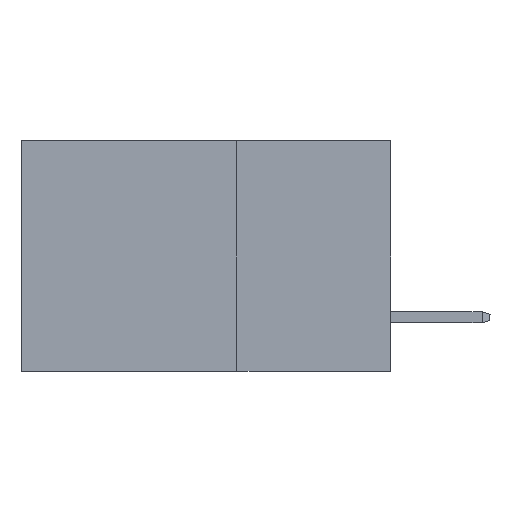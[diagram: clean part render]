
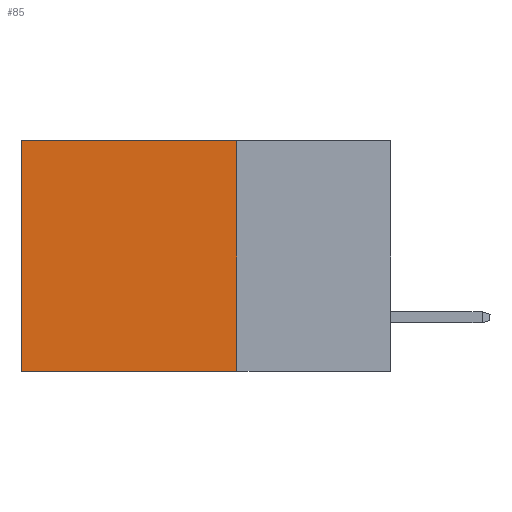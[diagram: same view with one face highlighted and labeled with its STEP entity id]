
A CAD part, left-side view. The second image highlights one B-rep face of the part: STEP entity #85.
In plain terms, the highlighted planar face has unit normal (-1, 0, 0).
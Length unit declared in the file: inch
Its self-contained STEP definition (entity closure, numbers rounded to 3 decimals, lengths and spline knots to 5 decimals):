
#85 = ADVANCED_FACE ( 'NONE', ( #702 ), #11993, .F. ) ;
#434 = VECTOR ( 'NONE', #9236, 39.37008 ) ;
#549 = ORIENTED_EDGE ( 'NONE', *, *, #10817, .F. ) ;
#702 = FACE_OUTER_BOUND ( 'NONE', #3182, .T. ) ;
#765 = ORIENTED_EDGE ( 'NONE', *, *, #3437, .F. ) ;
#810 = LINE ( 'NONE', #1016, #434 ) ;
#1016 = CARTESIAN_POINT ( 'NONE',  ( 0.2875, 0.6, -0.375 ) ) ;
#1050 = EDGE_CURVE ( 'NONE', #3864, #2768, #9512, .T. ) ;
#2768 = VERTEX_POINT ( 'NONE', #12126 ) ;
#3182 = EDGE_LOOP ( 'NONE', ( #14502, #549, #765, #5320 ) ) ;
#3437 = EDGE_CURVE ( 'NONE', #3864, #8057, #5598, .T. ) ;
#3864 = VERTEX_POINT ( 'NONE', #7282 ) ;
#5320 = ORIENTED_EDGE ( 'NONE', *, *, #1050, .T. ) ;
#5343 = EDGE_CURVE ( 'NONE', #2768, #10095, #810, .T. ) ;
#5598 = LINE ( 'NONE', #13385, #8169 ) ;
#6017 = DIRECTION ( 'NONE',  ( 0., 0., -1. ) ) ;
#6789 = CARTESIAN_POINT ( 'NONE',  ( 0.2875, 0.6, -0.375 ) ) ;
#7028 = CARTESIAN_POINT ( 'NONE',  ( 0.2875, 0.25, -0.375 ) ) ;
#7282 = CARTESIAN_POINT ( 'NONE',  ( 0.2875, 0.25, 0. ) ) ;
#7351 = VECTOR ( 'NONE', #8537, 39.37008 ) ;
#8057 = VERTEX_POINT ( 'NONE', #7028 ) ;
#8169 = VECTOR ( 'NONE', #13486, 39.37008 ) ;
#8257 = VECTOR ( 'NONE', #13772, 39.37008 ) ;
#8514 = CARTESIAN_POINT ( 'NONE',  ( 0.2875, 0.25, -0.375 ) ) ;
#8537 = DIRECTION ( 'NONE',  ( 0., 1., 0. ) ) ;
#8634 = CARTESIAN_POINT ( 'NONE',  ( 0.2875, 0.25, -0.375 ) ) ;
#9236 = DIRECTION ( 'NONE',  ( 0., 0., -1. ) ) ;
#9512 = LINE ( 'NONE', #11329, #8257 ) ;
#10095 = VERTEX_POINT ( 'NONE', #6789 ) ;
#10643 = DIRECTION ( 'NONE',  ( 1., 0., 0. ) ) ;
#10817 = EDGE_CURVE ( 'NONE', #8057, #10095, #12444, .T. ) ;
#11329 = CARTESIAN_POINT ( 'NONE',  ( 0.2875, 0.25, 0. ) ) ;
#11993 = PLANE ( 'NONE',  #14914 ) ;
#12126 = CARTESIAN_POINT ( 'NONE',  ( 0.2875, 0.6, 0. ) ) ;
#12444 = LINE ( 'NONE', #8634, #7351 ) ;
#13385 = CARTESIAN_POINT ( 'NONE',  ( 0.2875, 0.25, -0.375 ) ) ;
#13486 = DIRECTION ( 'NONE',  ( 0., 0., -1. ) ) ;
#13772 = DIRECTION ( 'NONE',  ( 0., 1., 0. ) ) ;
#14502 = ORIENTED_EDGE ( 'NONE', *, *, #5343, .T. ) ;
#14914 = AXIS2_PLACEMENT_3D ( 'NONE', #8514, #10643, #6017 ) ;
